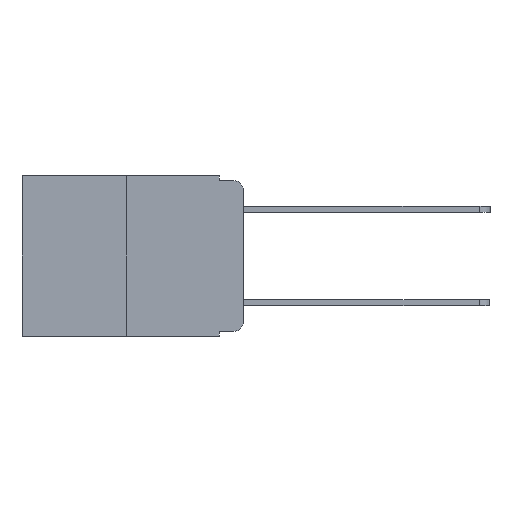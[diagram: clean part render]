
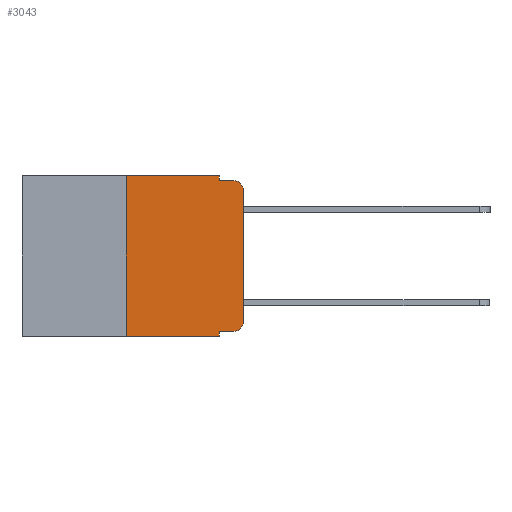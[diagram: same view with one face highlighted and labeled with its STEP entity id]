
A CAD part, left-side view. The second image highlights one B-rep face of the part: STEP entity #3043.
In plain terms, the highlighted planar face has unit normal (-1, 0, 0).
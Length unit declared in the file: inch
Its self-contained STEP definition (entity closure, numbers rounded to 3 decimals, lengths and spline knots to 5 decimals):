
#87 = CARTESIAN_POINT ( 'NONE',  ( 0., 0., -0.03 ) ) ;
#348 = VERTEX_POINT ( 'NONE', #5286 ) ;
#832 = DIRECTION ( 'NONE',  ( 0., -1., 0. ) ) ;
#864 = EDGE_CURVE ( 'NONE', #10644, #5014, #10524, .T. ) ;
#958 = EDGE_CURVE ( 'NONE', #3184, #2819, #11486, .T. ) ;
#1024 = DIRECTION ( 'NONE',  ( -1., 0., 0. ) ) ;
#1086 = DIRECTION ( 'NONE',  ( -1., 0., 0. ) ) ;
#1194 = CIRCLE ( 'NONE', #10299, 0.02 ) ;
#1498 = CARTESIAN_POINT ( 'NONE',  ( 0., 0., 0. ) ) ;
#1655 = LINE ( 'NONE', #10225, #6899 ) ;
#1667 = CARTESIAN_POINT ( 'NONE',  ( 0., 0.051, -0.343 ) ) ;
#1942 = DIRECTION ( 'NONE',  ( 0., -1., 0. ) ) ;
#2003 = EDGE_CURVE ( 'NONE', #348, #9439, #5751, .T. ) ;
#2033 = EDGE_LOOP ( 'NONE', ( #4637, #4370, #9885, #12888, #10444, #12593, #12260, #4707, #5609, #5321 ) ) ;
#2532 = FACE_OUTER_BOUND ( 'NONE', #2033, .T. ) ;
#2819 = VERTEX_POINT ( 'NONE', #87 ) ;
#2848 = CARTESIAN_POINT ( 'NONE',  ( 0., 0.051, -0.333 ) ) ;
#3043 = ADVANCED_FACE ( 'NONE', ( #2532 ), #11778, .F. ) ;
#3184 = VERTEX_POINT ( 'NONE', #12933 ) ;
#3185 = DIRECTION ( 'NONE',  ( 0., -1., 0. ) ) ;
#3633 = VECTOR ( 'NONE', #10745, 39.37008 ) ;
#3768 = DIRECTION ( 'NONE',  ( 0., 0., -1. ) ) ;
#3858 = CARTESIAN_POINT ( 'NONE',  ( 0., 0.25, 0. ) ) ;
#3920 = VERTEX_POINT ( 'NONE', #10213 ) ;
#4183 = CARTESIAN_POINT ( 'NONE',  ( 0., 0.051, -0.01 ) ) ;
#4370 = ORIENTED_EDGE ( 'NONE', *, *, #10842, .T. ) ;
#4537 = CIRCLE ( 'NONE', #12852, 0.02 ) ;
#4637 = ORIENTED_EDGE ( 'NONE', *, *, #958, .T. ) ;
#4707 = ORIENTED_EDGE ( 'NONE', *, *, #6521, .F. ) ;
#4917 = VECTOR ( 'NONE', #3768, 39.37008 ) ;
#5014 = VERTEX_POINT ( 'NONE', #1667 ) ;
#5047 = CARTESIAN_POINT ( 'NONE',  ( 0., 0.02, -0.333 ) ) ;
#5067 = CARTESIAN_POINT ( 'NONE',  ( 0., 0.051, 0. ) ) ;
#5217 = CARTESIAN_POINT ( 'NONE',  ( 0., 0.051, 0. ) ) ;
#5286 = CARTESIAN_POINT ( 'NONE',  ( 0., 0.051, -0.333 ) ) ;
#5321 = ORIENTED_EDGE ( 'NONE', *, *, #12261, .T. ) ;
#5405 = DIRECTION ( 'NONE',  ( 0., -1., 0. ) ) ;
#5438 = LINE ( 'NONE', #8434, #7825 ) ;
#5609 = ORIENTED_EDGE ( 'NONE', *, *, #2003, .T. ) ;
#5699 = VECTOR ( 'NONE', #11812, 39.37008 ) ;
#5751 = LINE ( 'NONE', #2848, #10487 ) ;
#6047 = LINE ( 'NONE', #5217, #5699 ) ;
#6323 = DIRECTION ( 'NONE',  ( 1., 0., 0. ) ) ;
#6521 = EDGE_CURVE ( 'NONE', #348, #5014, #11877, .T. ) ;
#6579 = LINE ( 'NONE', #3858, #3633 ) ;
#6583 = VERTEX_POINT ( 'NONE', #5067 ) ;
#6899 = VECTOR ( 'NONE', #5405, 39.37008 ) ;
#7205 = EDGE_CURVE ( 'NONE', #10644, #3920, #6579, .T. ) ;
#7412 = CARTESIAN_POINT ( 'NONE',  ( 0., 0.02, -0.01 ) ) ;
#7592 = CARTESIAN_POINT ( 'NONE',  ( 0., 0.02, -0.03 ) ) ;
#7645 = CARTESIAN_POINT ( 'NONE',  ( 0., 0.02, -0.313 ) ) ;
#7825 = VECTOR ( 'NONE', #3185, 39.37008 ) ;
#8434 = CARTESIAN_POINT ( 'NONE',  ( 0., 0.051, -0.01 ) ) ;
#8450 = EDGE_CURVE ( 'NONE', #6583, #12914, #6047, .T. ) ;
#8536 = DIRECTION ( 'NONE',  ( 0., 0., -1. ) ) ;
#8598 = DIRECTION ( 'NONE',  ( 0., 0., -1. ) ) ;
#9154 = CARTESIAN_POINT ( 'NONE',  ( 0., 0.25, -0.343 ) ) ;
#9406 = VECTOR ( 'NONE', #11299, 39.37008 ) ;
#9439 = VERTEX_POINT ( 'NONE', #5047 ) ;
#9779 = CARTESIAN_POINT ( 'NONE',  ( 0., 0.051, 0. ) ) ;
#9885 = ORIENTED_EDGE ( 'NONE', *, *, #10240, .F. ) ;
#10213 = CARTESIAN_POINT ( 'NONE',  ( 0., 0.25, 0. ) ) ;
#10225 = CARTESIAN_POINT ( 'NONE',  ( 0., 0.473, 0. ) ) ;
#10240 = EDGE_CURVE ( 'NONE', #12914, #12940, #5438, .T. ) ;
#10299 = AXIS2_PLACEMENT_3D ( 'NONE', #7592, #1024, #8536 ) ;
#10444 = ORIENTED_EDGE ( 'NONE', *, *, #13040, .F. ) ;
#10487 = VECTOR ( 'NONE', #1942, 39.37008 ) ;
#10524 = LINE ( 'NONE', #11478, #11066 ) ;
#10644 = VERTEX_POINT ( 'NONE', #9154 ) ;
#10745 = DIRECTION ( 'NONE',  ( 0., 0., 1. ) ) ;
#10804 = AXIS2_PLACEMENT_3D ( 'NONE', #11819, #6323, #12736 ) ;
#10842 = EDGE_CURVE ( 'NONE', #2819, #12940, #1194, .T. ) ;
#11066 = VECTOR ( 'NONE', #832, 39.37008 ) ;
#11299 = DIRECTION ( 'NONE',  ( 0., 0., 1. ) ) ;
#11478 = CARTESIAN_POINT ( 'NONE',  ( 0., 0.473, -0.343 ) ) ;
#11486 = LINE ( 'NONE', #1498, #9406 ) ;
#11778 = PLANE ( 'NONE',  #10804 ) ;
#11812 = DIRECTION ( 'NONE',  ( 0., 0., -1. ) ) ;
#11819 = CARTESIAN_POINT ( 'NONE',  ( 0., 0.473, 0. ) ) ;
#11877 = LINE ( 'NONE', #9779, #4917 ) ;
#12260 = ORIENTED_EDGE ( 'NONE', *, *, #864, .T. ) ;
#12261 = EDGE_CURVE ( 'NONE', #9439, #3184, #4537, .T. ) ;
#12593 = ORIENTED_EDGE ( 'NONE', *, *, #7205, .F. ) ;
#12736 = DIRECTION ( 'NONE',  ( 0., 0., -1. ) ) ;
#12852 = AXIS2_PLACEMENT_3D ( 'NONE', #7645, #1086, #8598 ) ;
#12888 = ORIENTED_EDGE ( 'NONE', *, *, #8450, .F. ) ;
#12914 = VERTEX_POINT ( 'NONE', #4183 ) ;
#12933 = CARTESIAN_POINT ( 'NONE',  ( 0., 0., -0.313 ) ) ;
#12940 = VERTEX_POINT ( 'NONE', #7412 ) ;
#13040 = EDGE_CURVE ( 'NONE', #3920, #6583, #1655, .T. ) ;
